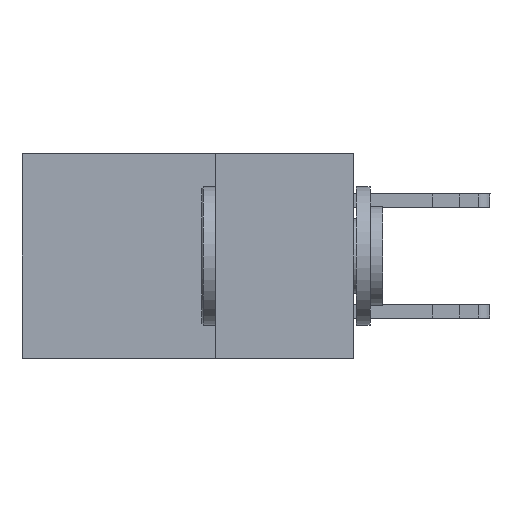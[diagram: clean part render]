
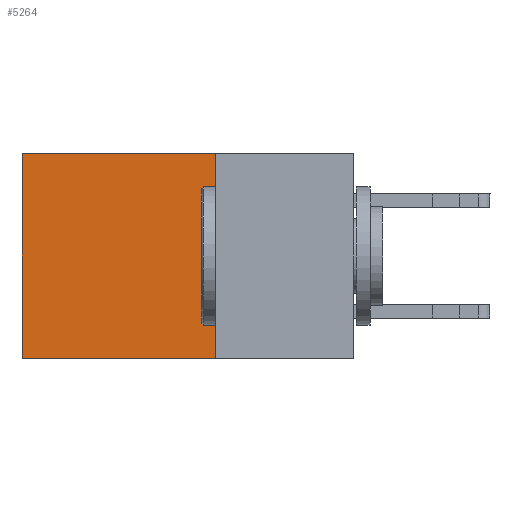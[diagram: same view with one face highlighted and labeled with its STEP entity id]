
A CAD part, left-side view. The second image highlights one B-rep face of the part: STEP entity #5264.
In plain terms, the highlighted planar face has unit normal (-1, 0, 0).
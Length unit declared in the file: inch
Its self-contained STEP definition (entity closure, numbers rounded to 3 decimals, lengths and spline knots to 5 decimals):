
#130 = DIRECTION ( 'NONE',  ( 1., 0., 0. ) ) ;
#1595 = DIRECTION ( 'NONE',  ( 0., 1., 0. ) ) ;
#2122 = EDGE_CURVE ( 'NONE', #8059, #2151, #17731, .T. ) ;
#2151 = VERTEX_POINT ( 'NONE', #9625 ) ;
#2315 = LINE ( 'NONE', #18017, #11246 ) ;
#2634 = EDGE_CURVE ( 'NONE', #17614, #13301, #10005, .T. ) ;
#2806 = ORIENTED_EDGE ( 'NONE', *, *, #9015, .T. ) ;
#2932 = VECTOR ( 'NONE', #18243, 39.37008 ) ;
#3283 = PLANE ( 'NONE',  #18482 ) ;
#3764 = DIRECTION ( 'NONE',  ( 0., 1., 0. ) ) ;
#4552 = VECTOR ( 'NONE', #1595, 39.37008 ) ;
#4823 = LINE ( 'NONE', #15846, #4552 ) ;
#4936 = DIRECTION ( 'NONE',  ( 0., 0., -1. ) ) ;
#5026 = DIRECTION ( 'NONE',  ( 0., 0., -1. ) ) ;
#5264 = ADVANCED_FACE ( 'NONE', ( #19391 ), #3283, .F. ) ;
#5296 = ORIENTED_EDGE ( 'NONE', *, *, #2122, .F. ) ;
#8059 = VERTEX_POINT ( 'NONE', #19727 ) ;
#8071 = VECTOR ( 'NONE', #4936, 39.37008 ) ;
#8448 = CARTESIAN_POINT ( 'NONE',  ( 0.2875, 0.6, 0. ) ) ;
#8475 = CARTESIAN_POINT ( 'NONE',  ( 0.2875, 0.6, 0. ) ) ;
#9015 = EDGE_CURVE ( 'NONE', #8059, #17614, #2315, .T. ) ;
#9625 = CARTESIAN_POINT ( 'NONE',  ( 0.2875, 0.25, -0.37 ) ) ;
#9994 = ORIENTED_EDGE ( 'NONE', *, *, #2634, .T. ) ;
#10005 = LINE ( 'NONE', #8448, #2932 ) ;
#11179 = CARTESIAN_POINT ( 'NONE',  ( 0.2875, 0.25, 0. ) ) ;
#11246 = VECTOR ( 'NONE', #3764, 39.37008 ) ;
#11473 = CARTESIAN_POINT ( 'NONE',  ( 0.2875, 0.25, 0. ) ) ;
#12944 = EDGE_LOOP ( 'NONE', ( #9994, #15191, #5296, #2806 ) ) ;
#13301 = VERTEX_POINT ( 'NONE', #20078 ) ;
#14393 = EDGE_CURVE ( 'NONE', #2151, #13301, #4823, .T. ) ;
#15191 = ORIENTED_EDGE ( 'NONE', *, *, #14393, .F. ) ;
#15846 = CARTESIAN_POINT ( 'NONE',  ( 0.2875, 0.25, -0.37 ) ) ;
#17614 = VERTEX_POINT ( 'NONE', #8475 ) ;
#17731 = LINE ( 'NONE', #11179, #8071 ) ;
#18017 = CARTESIAN_POINT ( 'NONE',  ( 0.2875, 0.25, 0. ) ) ;
#18243 = DIRECTION ( 'NONE',  ( 0., 0., -1. ) ) ;
#18482 = AXIS2_PLACEMENT_3D ( 'NONE', #11473, #130, #5026 ) ;
#19391 = FACE_OUTER_BOUND ( 'NONE', #12944, .T. ) ;
#19727 = CARTESIAN_POINT ( 'NONE',  ( 0.2875, 0.25, 0. ) ) ;
#20078 = CARTESIAN_POINT ( 'NONE',  ( 0.2875, 0.6, -0.37 ) ) ;
